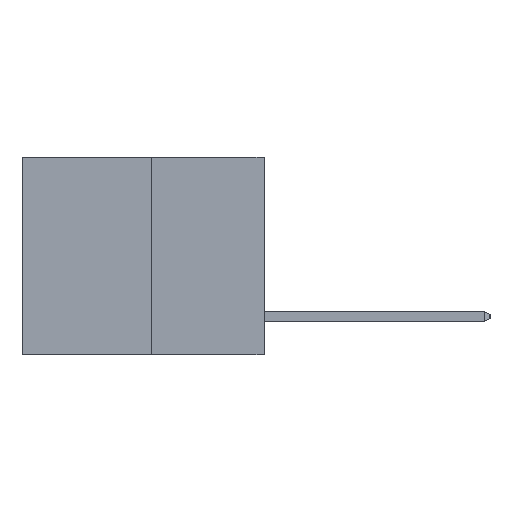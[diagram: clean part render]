
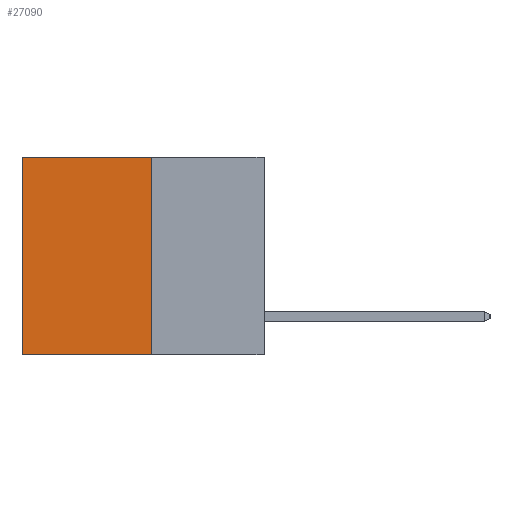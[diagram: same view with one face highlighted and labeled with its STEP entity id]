
A CAD part, left-side view. The second image highlights one B-rep face of the part: STEP entity #27090.
In plain terms, the highlighted planar face has unit normal (-1, 0, 0).
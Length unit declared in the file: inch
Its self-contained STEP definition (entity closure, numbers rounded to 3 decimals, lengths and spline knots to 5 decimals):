
#1552 = ORIENTED_EDGE ( 'NONE', *, *, #12107, .F. ) ;
#2108 = LINE ( 'NONE', #4860, #26598 ) ;
#2428 = CARTESIAN_POINT ( 'NONE',  ( 0.3165, 0.6, 0. ) ) ;
#2985 = DIRECTION ( 'NONE',  ( 0., 1., 0. ) ) ;
#3845 = DIRECTION ( 'NONE',  ( 1., 0., 0. ) ) ;
#4233 = VECTOR ( 'NONE', #2985, 39.37008 ) ;
#4397 = VERTEX_POINT ( 'NONE', #9008 ) ;
#4581 = FACE_OUTER_BOUND ( 'NONE', #15993, .T. ) ;
#4860 = CARTESIAN_POINT ( 'NONE',  ( 0.3165, 0.6, -0.49 ) ) ;
#4970 = AXIS2_PLACEMENT_3D ( 'NONE', #22645, #3845, #27396 ) ;
#5687 = VECTOR ( 'NONE', #22509, 39.37008 ) ;
#5893 = ORIENTED_EDGE ( 'NONE', *, *, #8091, .T. ) ;
#7227 = PLANE ( 'NONE',  #4970 ) ;
#8091 = EDGE_CURVE ( 'NONE', #27255, #20329, #2108, .T. ) ;
#8944 = ORIENTED_EDGE ( 'NONE', *, *, #18492, .F. ) ;
#9008 = CARTESIAN_POINT ( 'NONE',  ( 0.3165, 0.28, -0.49 ) ) ;
#11288 = EDGE_CURVE ( 'NONE', #22142, #27255, #11518, .T. ) ;
#11395 = CARTESIAN_POINT ( 'NONE',  ( 0.3165, 0.6, -0.49 ) ) ;
#11518 = LINE ( 'NONE', #24353, #5687 ) ;
#11909 = LINE ( 'NONE', #19399, #13310 ) ;
#12107 = EDGE_CURVE ( 'NONE', #4397, #20329, #24549, .T. ) ;
#12767 = ORIENTED_EDGE ( 'NONE', *, *, #11288, .T. ) ;
#13310 = VECTOR ( 'NONE', #15282, 39.37008 ) ;
#14799 = CARTESIAN_POINT ( 'NONE',  ( 0.3165, 0.28, 0. ) ) ;
#15282 = DIRECTION ( 'NONE',  ( 0., 0., -1. ) ) ;
#15993 = EDGE_LOOP ( 'NONE', ( #5893, #1552, #8944, #12767 ) ) ;
#16205 = CARTESIAN_POINT ( 'NONE',  ( 0.3165, 0.28, -0.49 ) ) ;
#18492 = EDGE_CURVE ( 'NONE', #22142, #4397, #11909, .T. ) ;
#19399 = CARTESIAN_POINT ( 'NONE',  ( 0.3165, 0.28, -0.49 ) ) ;
#20329 = VERTEX_POINT ( 'NONE', #11395 ) ;
#22142 = VERTEX_POINT ( 'NONE', #14799 ) ;
#22483 = DIRECTION ( 'NONE',  ( 0., 0., -1. ) ) ;
#22509 = DIRECTION ( 'NONE',  ( 0., 1., 0. ) ) ;
#22645 = CARTESIAN_POINT ( 'NONE',  ( 0.3165, 0.28, -0.49 ) ) ;
#24353 = CARTESIAN_POINT ( 'NONE',  ( 0.3165, 0.28, 0. ) ) ;
#24549 = LINE ( 'NONE', #16205, #4233 ) ;
#26598 = VECTOR ( 'NONE', #22483, 39.37008 ) ;
#27090 = ADVANCED_FACE ( 'NONE', ( #4581 ), #7227, .F. ) ;
#27255 = VERTEX_POINT ( 'NONE', #2428 ) ;
#27396 = DIRECTION ( 'NONE',  ( 0., 0., -1. ) ) ;
